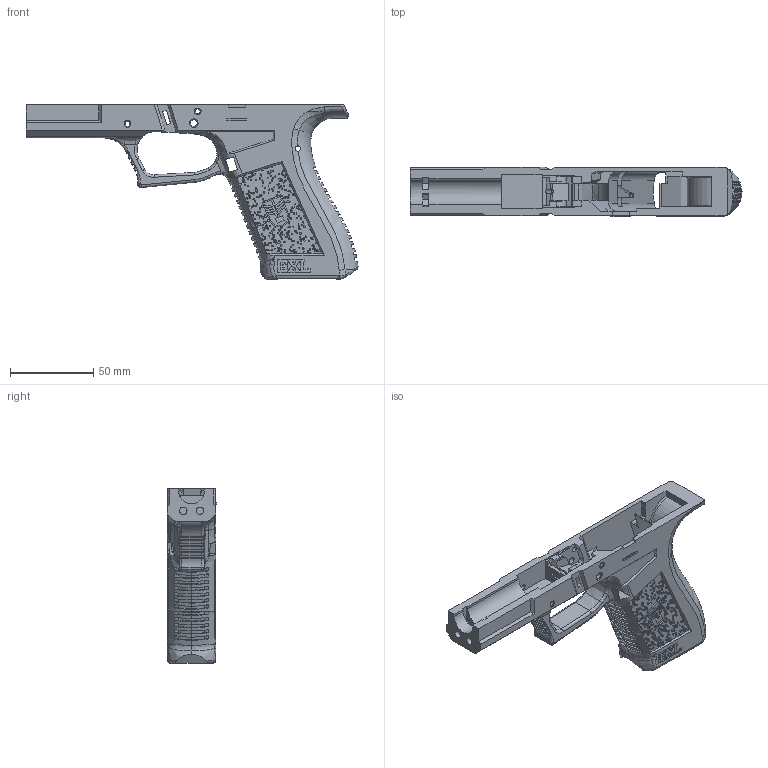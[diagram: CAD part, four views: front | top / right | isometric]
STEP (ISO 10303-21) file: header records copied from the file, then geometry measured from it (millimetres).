
FILE_DESCRIPTION(/* description */ (''),/* implementation_level */ '2;1');
FILE_NAME(/* name */ 'DD17.2 CRUSHER17.step',/* time_stamp */ '2022-08-30T18:43:14-05:00',/* author */ (''),/* organization */ (''),/* preprocessor_version */ 'ST-DEVELOPER v19',/* originating_system */ 'Autodesk Translation Framework v11.7.0.108',/* authorisation */ '');
FILE_SCHEMA (('AUTOMOTIVE_DESIGN { 1 0 10303 214 3 1 1 }'));
Products named in the file (1): DD17.2 SDI GXL CRUSHER
Bounding box: 199.66 x 29.73 x 104.95 mm (x, y, z)
Volume: 108605.2 mm3; surface area: 52629.2 mm2
Topology: 1 solids, 2 shells, 3391 faces, 8890 edges, 5883 vertices
Faces by surface type: bspline 2281, plane 1035, cylinder 64, torus 11
Full cylindrical faces by diameter (mm): 1.933 x1, 3 x4, 3.2 x2, 3.5 x1, 4.1 x2, 4.5 x2
Entity records: 136975 total; most frequent: CARTESIAN_POINT 75692, ORIENTED_EDGE 17762, EDGE_CURVE 8881, DIRECTION 6356, VERTEX_POINT 5883, EDGE_LOOP 3814, LINE 3632, VECTOR 3632
